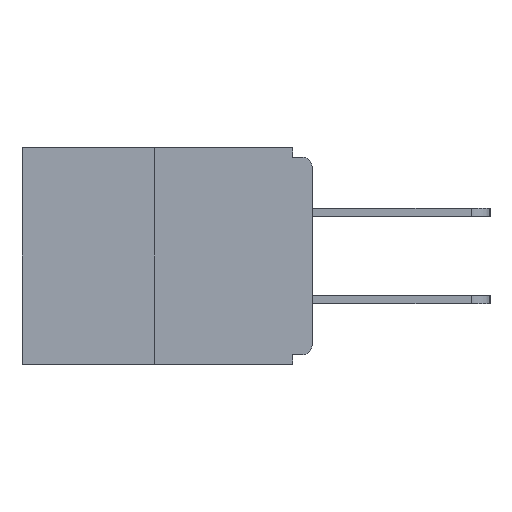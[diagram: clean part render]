
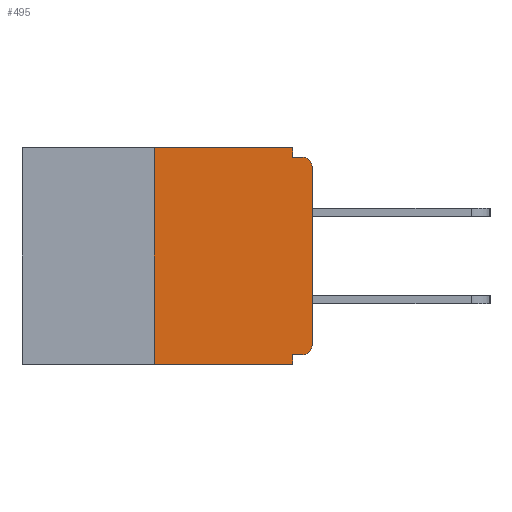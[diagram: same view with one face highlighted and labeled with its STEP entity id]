
A CAD part, left-side view. The second image highlights one B-rep face of the part: STEP entity #495.
In plain terms, the highlighted planar face has unit normal (-1, 0, 0).
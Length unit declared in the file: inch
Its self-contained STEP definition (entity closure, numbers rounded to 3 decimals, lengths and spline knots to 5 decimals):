
#165 = EDGE_CURVE ( 'NONE', #3558, #12955, #9483, .T. ) ;
#437 = CARTESIAN_POINT ( 'NONE',  ( 0., 0.25, 0. ) ) ;
#462 = CARTESIAN_POINT ( 'NONE',  ( 0., 0.015, -0.313 ) ) ;
#495 = ADVANCED_FACE ( 'NONE', ( #4521 ), #3742, .F. ) ;
#930 = LINE ( 'NONE', #437, #8774 ) ;
#1260 = LINE ( 'NONE', #13147, #2354 ) ;
#1418 = CARTESIAN_POINT ( 'NONE',  ( 0., 0.031, 0. ) ) ;
#1615 = CARTESIAN_POINT ( 'NONE',  ( 0., 0.25, -0.343 ) ) ;
#1801 = VECTOR ( 'NONE', #2241, 39.37008 ) ;
#1837 = LINE ( 'NONE', #12270, #7297 ) ;
#1881 = DIRECTION ( 'NONE',  ( 0., 1., 0. ) ) ;
#2064 = ORIENTED_EDGE ( 'NONE', *, *, #6136, .T. ) ;
#2241 = DIRECTION ( 'NONE',  ( 0., 0., -1. ) ) ;
#2297 = EDGE_CURVE ( 'NONE', #8964, #9349, #930, .T. ) ;
#2354 = VECTOR ( 'NONE', #7114, 39.37008 ) ;
#2514 = LINE ( 'NONE', #11474, #13071 ) ;
#2670 = LINE ( 'NONE', #9878, #13223 ) ;
#2705 = CARTESIAN_POINT ( 'NONE',  ( 0., 0.015, -0.015 ) ) ;
#2973 = ORIENTED_EDGE ( 'NONE', *, *, #9271, .T. ) ;
#3108 = CARTESIAN_POINT ( 'NONE',  ( 0., 0., 0. ) ) ;
#3315 = VERTEX_POINT ( 'NONE', #8014 ) ;
#3457 = VECTOR ( 'NONE', #10261, 39.37008 ) ;
#3531 = DIRECTION ( 'NONE',  ( 0., 0., 1. ) ) ;
#3558 = VERTEX_POINT ( 'NONE', #11713 ) ;
#3561 = DIRECTION ( 'NONE',  ( -1., 0., 0. ) ) ;
#3596 = EDGE_CURVE ( 'NONE', #11360, #3558, #8307, .T. ) ;
#3742 = PLANE ( 'NONE',  #10523 ) ;
#4200 = VECTOR ( 'NONE', #12355, 39.37008 ) ;
#4521 = FACE_OUTER_BOUND ( 'NONE', #10553, .T. ) ;
#4724 = VERTEX_POINT ( 'NONE', #11282 ) ;
#4774 = DIRECTION ( 'NONE',  ( 1., 0., 0. ) ) ;
#4909 = EDGE_CURVE ( 'NONE', #4724, #9586, #8037, .T. ) ;
#4928 = ORIENTED_EDGE ( 'NONE', *, *, #3596, .T. ) ;
#5360 = ORIENTED_EDGE ( 'NONE', *, *, #6486, .F. ) ;
#5412 = DIRECTION ( 'NONE',  ( -1., 0., 0. ) ) ;
#6136 = EDGE_CURVE ( 'NONE', #12955, #9083, #9273, .T. ) ;
#6486 = EDGE_CURVE ( 'NONE', #9349, #7182, #1260, .T. ) ;
#7001 = LINE ( 'NONE', #10177, #3457 ) ;
#7008 = EDGE_CURVE ( 'NONE', #11360, #4724, #2670, .T. ) ;
#7114 = DIRECTION ( 'NONE',  ( 0., -1., 0. ) ) ;
#7182 = VERTEX_POINT ( 'NONE', #1418 ) ;
#7190 = CARTESIAN_POINT ( 'NONE',  ( 0., 0.25, 0. ) ) ;
#7208 = ORIENTED_EDGE ( 'NONE', *, *, #2297, .F. ) ;
#7297 = VECTOR ( 'NONE', #8336, 39.37008 ) ;
#7374 = CARTESIAN_POINT ( 'NONE',  ( 0., 0.031, -0.343 ) ) ;
#7567 = EDGE_CURVE ( 'NONE', #7182, #3315, #2514, .T. ) ;
#7847 = DIRECTION ( 'NONE',  ( 0., 0., -1. ) ) ;
#8014 = CARTESIAN_POINT ( 'NONE',  ( 0., 0.031, -0.015 ) ) ;
#8037 = LINE ( 'NONE', #7374, #1801 ) ;
#8198 = ORIENTED_EDGE ( 'NONE', *, *, #165, .T. ) ;
#8205 = CARTESIAN_POINT ( 'NONE',  ( 0., 0.015, -0.328 ) ) ;
#8307 = CIRCLE ( 'NONE', #13247, 0.015 ) ;
#8336 = DIRECTION ( 'NONE',  ( 0., -1., 0. ) ) ;
#8354 = ORIENTED_EDGE ( 'NONE', *, *, #4909, .F. ) ;
#8599 = ORIENTED_EDGE ( 'NONE', *, *, #7567, .F. ) ;
#8774 = VECTOR ( 'NONE', #3531, 39.37008 ) ;
#8964 = VERTEX_POINT ( 'NONE', #1615 ) ;
#9083 = VERTEX_POINT ( 'NONE', #2705 ) ;
#9271 = EDGE_CURVE ( 'NONE', #8964, #9586, #1837, .T. ) ;
#9273 = CIRCLE ( 'NONE', #11811, 0.015 ) ;
#9349 = VERTEX_POINT ( 'NONE', #7190 ) ;
#9353 = DIRECTION ( 'NONE',  ( 0., 0., -1. ) ) ;
#9483 = LINE ( 'NONE', #3108, #4200 ) ;
#9586 = VERTEX_POINT ( 'NONE', #10640 ) ;
#9602 = CARTESIAN_POINT ( 'NONE',  ( 0., 0.015, -0.03 ) ) ;
#9759 = CARTESIAN_POINT ( 'NONE',  ( 0., 0., -0.03 ) ) ;
#9878 = CARTESIAN_POINT ( 'NONE',  ( 0., 0., -0.328 ) ) ;
#10177 = CARTESIAN_POINT ( 'NONE',  ( 0., 0., -0.015 ) ) ;
#10201 = ORIENTED_EDGE ( 'NONE', *, *, #11869, .F. ) ;
#10261 = DIRECTION ( 'NONE',  ( 0., -1., 0. ) ) ;
#10510 = DIRECTION ( 'NONE',  ( 0., 0., -1. ) ) ;
#10523 = AXIS2_PLACEMENT_3D ( 'NONE', #11841, #4774, #7847 ) ;
#10553 = EDGE_LOOP ( 'NONE', ( #5360, #7208, #2973, #8354, #12513, #4928, #8198, #2064, #10201, #8599 ) ) ;
#10640 = CARTESIAN_POINT ( 'NONE',  ( 0., 0.031, -0.343 ) ) ;
#10733 = DIRECTION ( 'NONE',  ( 0., 0., -1. ) ) ;
#11282 = CARTESIAN_POINT ( 'NONE',  ( 0., 0.031, -0.328 ) ) ;
#11360 = VERTEX_POINT ( 'NONE', #8205 ) ;
#11474 = CARTESIAN_POINT ( 'NONE',  ( 0., 0.031, 0. ) ) ;
#11713 = CARTESIAN_POINT ( 'NONE',  ( 0., 0., -0.313 ) ) ;
#11811 = AXIS2_PLACEMENT_3D ( 'NONE', #9602, #5412, #10510 ) ;
#11841 = CARTESIAN_POINT ( 'NONE',  ( 0., 0.46, 0. ) ) ;
#11869 = EDGE_CURVE ( 'NONE', #3315, #9083, #7001, .T. ) ;
#12270 = CARTESIAN_POINT ( 'NONE',  ( 0., 0.46, -0.343 ) ) ;
#12355 = DIRECTION ( 'NONE',  ( 0., 0., 1. ) ) ;
#12513 = ORIENTED_EDGE ( 'NONE', *, *, #7008, .F. ) ;
#12955 = VERTEX_POINT ( 'NONE', #9759 ) ;
#13071 = VECTOR ( 'NONE', #9353, 39.37008 ) ;
#13147 = CARTESIAN_POINT ( 'NONE',  ( 0., 0.46, 0. ) ) ;
#13223 = VECTOR ( 'NONE', #1881, 39.37008 ) ;
#13247 = AXIS2_PLACEMENT_3D ( 'NONE', #462, #3561, #10733 ) ;
